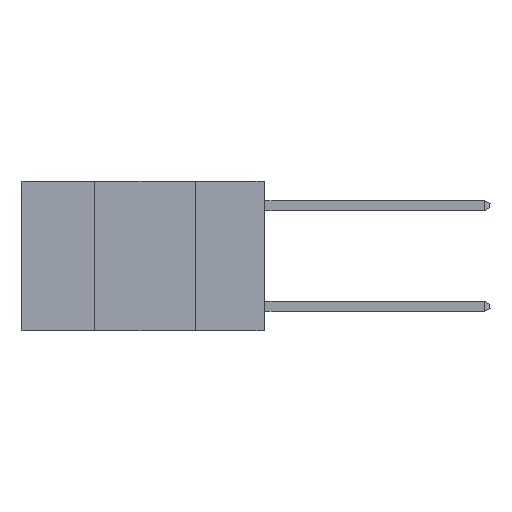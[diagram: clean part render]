
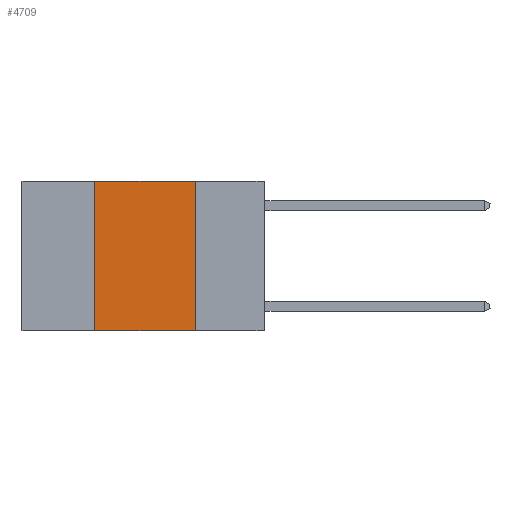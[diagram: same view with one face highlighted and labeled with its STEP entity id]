
A CAD part, left-side view. The second image highlights one B-rep face of the part: STEP entity #4709.
In plain terms, the highlighted planar face has unit normal (-1, 0, 0).
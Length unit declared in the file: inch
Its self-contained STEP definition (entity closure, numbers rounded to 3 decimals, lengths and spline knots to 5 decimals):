
#266 = LINE ( 'NONE', #10243, #12737 ) ;
#341 = DIRECTION ( 'NONE',  ( 0., 0., -1. ) ) ;
#459 = LINE ( 'NONE', #8149, #14788 ) ;
#814 = CARTESIAN_POINT ( 'NONE',  ( 0., 0.42, 0. ) ) ;
#1163 = DIRECTION ( 'NONE',  ( 0., 0., -1. ) ) ;
#1219 = CARTESIAN_POINT ( 'NONE',  ( 0., 0.17, 0. ) ) ;
#2042 = ORIENTED_EDGE ( 'NONE', *, *, #15100, .T. ) ;
#2418 = VERTEX_POINT ( 'NONE', #814 ) ;
#2551 = ORIENTED_EDGE ( 'NONE', *, *, #9902, .F. ) ;
#2717 = VERTEX_POINT ( 'NONE', #14799 ) ;
#3554 = PLANE ( 'NONE',  #15588 ) ;
#4709 = ADVANCED_FACE ( 'NONE', ( #14536 ), #3554, .F. ) ;
#4787 = DIRECTION ( 'NONE',  ( 0., 0., 1. ) ) ;
#5293 = EDGE_CURVE ( 'NONE', #11464, #2717, #266, .T. ) ;
#5728 = CARTESIAN_POINT ( 'NONE',  ( 0., 0.6, 0. ) ) ;
#5918 = EDGE_CURVE ( 'NONE', #2418, #11464, #12036, .T. ) ;
#5998 = ORIENTED_EDGE ( 'NONE', *, *, #5918, .F. ) ;
#6045 = VECTOR ( 'NONE', #4787, 39.37008 ) ;
#6146 = CARTESIAN_POINT ( 'NONE',  ( 0., 0.42, 0. ) ) ;
#6148 = VERTEX_POINT ( 'NONE', #13505 ) ;
#8149 = CARTESIAN_POINT ( 'NONE',  ( 0., 0.6, -0.37 ) ) ;
#8777 = DIRECTION ( 'NONE',  ( 1., 0., 0. ) ) ;
#8863 = CARTESIAN_POINT ( 'NONE',  ( 0., 0.6, 0. ) ) ;
#9902 = EDGE_CURVE ( 'NONE', #6148, #2418, #10723, .T. ) ;
#10243 = CARTESIAN_POINT ( 'NONE',  ( 0., 0.17, 0. ) ) ;
#10723 = LINE ( 'NONE', #6146, #6045 ) ;
#10821 = DIRECTION ( 'NONE',  ( 0., -1., 0. ) ) ;
#10932 = VECTOR ( 'NONE', #10821, 39.37008 ) ;
#11464 = VERTEX_POINT ( 'NONE', #1219 ) ;
#12036 = LINE ( 'NONE', #5728, #10932 ) ;
#12737 = VECTOR ( 'NONE', #341, 39.37008 ) ;
#12855 = ORIENTED_EDGE ( 'NONE', *, *, #5293, .F. ) ;
#13145 = EDGE_LOOP ( 'NONE', ( #12855, #5998, #2551, #2042 ) ) ;
#13505 = CARTESIAN_POINT ( 'NONE',  ( 0., 0.42, -0.37 ) ) ;
#14536 = FACE_OUTER_BOUND ( 'NONE', #13145, .T. ) ;
#14788 = VECTOR ( 'NONE', #15304, 39.37008 ) ;
#14799 = CARTESIAN_POINT ( 'NONE',  ( 0., 0.17, -0.37 ) ) ;
#15100 = EDGE_CURVE ( 'NONE', #6148, #2717, #459, .T. ) ;
#15304 = DIRECTION ( 'NONE',  ( 0., -1., 0. ) ) ;
#15588 = AXIS2_PLACEMENT_3D ( 'NONE', #8863, #8777, #1163 ) ;
